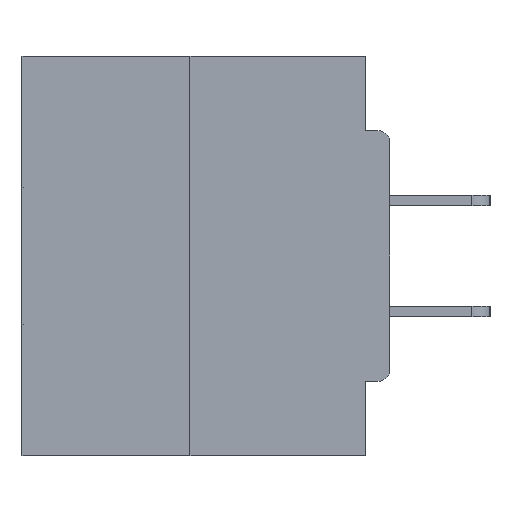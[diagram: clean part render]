
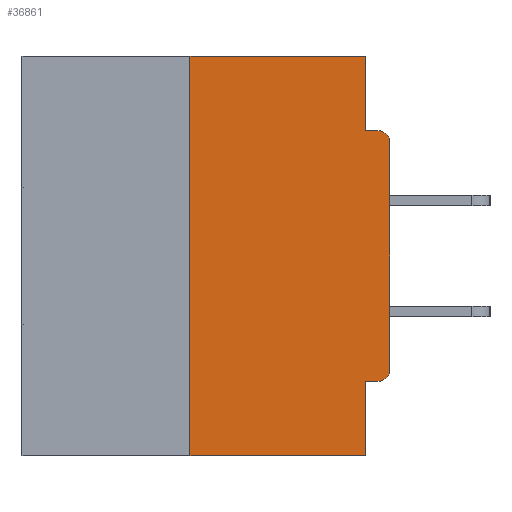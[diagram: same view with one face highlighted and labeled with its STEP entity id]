
A CAD part, left-side view. The second image highlights one B-rep face of the part: STEP entity #36861.
In plain terms, the highlighted planar face has unit normal (-1, 0, 0).
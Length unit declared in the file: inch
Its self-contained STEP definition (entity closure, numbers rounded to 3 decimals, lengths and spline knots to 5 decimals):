
#496 = VECTOR ( 'NONE', #21159, 39.37008 ) ;
#781 = ORIENTED_EDGE ( 'NONE', *, *, #27009, .T. ) ;
#1666 = CARTESIAN_POINT ( 'NONE',  ( 0., 0., 0. ) ) ;
#1993 = CARTESIAN_POINT ( 'NONE',  ( 0., 0.031, 0. ) ) ;
#3010 = VECTOR ( 'NONE', #34634, 39.37008 ) ;
#3475 = PLANE ( 'NONE',  #36398 ) ;
#3596 = AXIS2_PLACEMENT_3D ( 'NONE', #28553, #37429, #28154 ) ;
#4270 = ORIENTED_EDGE ( 'NONE', *, *, #21735, .F. ) ;
#4597 = CARTESIAN_POINT ( 'NONE',  ( 0., 0.031, -0.5 ) ) ;
#4950 = CARTESIAN_POINT ( 'NONE',  ( 0., 0.015, -0.1085 ) ) ;
#5114 = VERTEX_POINT ( 'NONE', #16531 ) ;
#5177 = ORIENTED_EDGE ( 'NONE', *, *, #6664, .F. ) ;
#6664 = EDGE_CURVE ( 'NONE', #37443, #7307, #17230, .T. ) ;
#6822 = DIRECTION ( 'NONE',  ( 0., 0., -1. ) ) ;
#7307 = VERTEX_POINT ( 'NONE', #33008 ) ;
#7712 = ORIENTED_EDGE ( 'NONE', *, *, #18043, .T. ) ;
#7819 = VECTOR ( 'NONE', #20376, 39.37008 ) ;
#7826 = AXIS2_PLACEMENT_3D ( 'NONE', #4950, #31469, #34625 ) ;
#8199 = CARTESIAN_POINT ( 'NONE',  ( 0., 0.25, 0. ) ) ;
#8890 = CARTESIAN_POINT ( 'NONE',  ( 0., 0., -0.0935 ) ) ;
#8992 = LINE ( 'NONE', #33144, #18639 ) ;
#9010 = EDGE_CURVE ( 'NONE', #9735, #37443, #37340, .T. ) ;
#9191 = CARTESIAN_POINT ( 'NONE',  ( 0., 0.46, 0. ) ) ;
#9397 = DIRECTION ( 'NONE',  ( 0., 0., -1. ) ) ;
#9735 = VERTEX_POINT ( 'NONE', #36093 ) ;
#10626 = DIRECTION ( 'NONE',  ( 0., 0., 1. ) ) ;
#10912 = ORIENTED_EDGE ( 'NONE', *, *, #15432, .T. ) ;
#11268 = CARTESIAN_POINT ( 'NONE',  ( 0., 0.46, -0.5 ) ) ;
#12174 = FACE_OUTER_BOUND ( 'NONE', #25087, .T. ) ;
#12441 = LINE ( 'NONE', #8890, #496 ) ;
#12648 = VERTEX_POINT ( 'NONE', #37939 ) ;
#13679 = VECTOR ( 'NONE', #32454, 39.37008 ) ;
#14622 = LINE ( 'NONE', #11268, #7819 ) ;
#14968 = EDGE_CURVE ( 'NONE', #12648, #33162, #8992, .T. ) ;
#15432 = EDGE_CURVE ( 'NONE', #26244, #21813, #21744, .T. ) ;
#15540 = VERTEX_POINT ( 'NONE', #32619 ) ;
#15544 = VERTEX_POINT ( 'NONE', #23908 ) ;
#15575 = CIRCLE ( 'NONE', #3596, 0.015 ) ;
#16531 = CARTESIAN_POINT ( 'NONE',  ( 0., 0.015, -0.4065 ) ) ;
#17198 = CARTESIAN_POINT ( 'NONE',  ( 0., 0.015, -0.0935 ) ) ;
#17230 = LINE ( 'NONE', #19623, #33528 ) ;
#18043 = EDGE_CURVE ( 'NONE', #5114, #15540, #15575, .T. ) ;
#18361 = ORIENTED_EDGE ( 'NONE', *, *, #9010, .F. ) ;
#18639 = VECTOR ( 'NONE', #6822, 39.37008 ) ;
#18725 = ORIENTED_EDGE ( 'NONE', *, *, #29654, .F. ) ;
#18946 = CARTESIAN_POINT ( 'NONE',  ( 0., 0.25, 0. ) ) ;
#19623 = CARTESIAN_POINT ( 'NONE',  ( 0., 0.46, 0. ) ) ;
#20376 = DIRECTION ( 'NONE',  ( 0., -1., 0. ) ) ;
#20426 = LINE ( 'NONE', #1666, #28159 ) ;
#21159 = DIRECTION ( 'NONE',  ( 0., -1., 0. ) ) ;
#21265 = ORIENTED_EDGE ( 'NONE', *, *, #28235, .T. ) ;
#21735 = EDGE_CURVE ( 'NONE', #7307, #15544, #29099, .T. ) ;
#21744 = CIRCLE ( 'NONE', #7826, 0.015 ) ;
#21813 = VERTEX_POINT ( 'NONE', #17198 ) ;
#23908 = CARTESIAN_POINT ( 'NONE',  ( 0., 0.031, -0.0935 ) ) ;
#25087 = EDGE_LOOP ( 'NONE', ( #5177, #18361, #781, #32816, #18725, #7712, #21265, #10912, #27222, #4270 ) ) ;
#26244 = VERTEX_POINT ( 'NONE', #30634 ) ;
#26517 = LINE ( 'NONE', #26708, #13679 ) ;
#26708 = CARTESIAN_POINT ( 'NONE',  ( 0., 0., -0.4065 ) ) ;
#27009 = EDGE_CURVE ( 'NONE', #9735, #33162, #14622, .T. ) ;
#27027 = DIRECTION ( 'NONE',  ( 1., 0., 0. ) ) ;
#27222 = ORIENTED_EDGE ( 'NONE', *, *, #31224, .F. ) ;
#28154 = DIRECTION ( 'NONE',  ( 0., 0., -1. ) ) ;
#28159 = VECTOR ( 'NONE', #34897, 39.37008 ) ;
#28235 = EDGE_CURVE ( 'NONE', #15540, #26244, #20426, .T. ) ;
#28553 = CARTESIAN_POINT ( 'NONE',  ( 0., 0.015, -0.3915 ) ) ;
#29099 = LINE ( 'NONE', #1993, #3010 ) ;
#29311 = DIRECTION ( 'NONE',  ( 0., -1., 0. ) ) ;
#29654 = EDGE_CURVE ( 'NONE', #5114, #12648, #26517, .T. ) ;
#30634 = CARTESIAN_POINT ( 'NONE',  ( 0., 0., -0.1085 ) ) ;
#31224 = EDGE_CURVE ( 'NONE', #15544, #21813, #12441, .T. ) ;
#31469 = DIRECTION ( 'NONE',  ( -1., 0., 0. ) ) ;
#32454 = DIRECTION ( 'NONE',  ( 0., 1., 0. ) ) ;
#32619 = CARTESIAN_POINT ( 'NONE',  ( 0., 0., -0.3915 ) ) ;
#32816 = ORIENTED_EDGE ( 'NONE', *, *, #14968, .F. ) ;
#33008 = CARTESIAN_POINT ( 'NONE',  ( 0., 0.031, 0. ) ) ;
#33144 = CARTESIAN_POINT ( 'NONE',  ( 0., 0.031, -0.5 ) ) ;
#33162 = VERTEX_POINT ( 'NONE', #4597 ) ;
#33528 = VECTOR ( 'NONE', #29311, 39.37008 ) ;
#34625 = DIRECTION ( 'NONE',  ( 0., 0., -1. ) ) ;
#34634 = DIRECTION ( 'NONE',  ( 0., 0., -1. ) ) ;
#34636 = VECTOR ( 'NONE', #10626, 39.37008 ) ;
#34897 = DIRECTION ( 'NONE',  ( 0., 0., 1. ) ) ;
#36093 = CARTESIAN_POINT ( 'NONE',  ( 0., 0.25, -0.5 ) ) ;
#36398 = AXIS2_PLACEMENT_3D ( 'NONE', #9191, #27027, #9397 ) ;
#36861 = ADVANCED_FACE ( 'NONE', ( #12174 ), #3475, .F. ) ;
#37340 = LINE ( 'NONE', #18946, #34636 ) ;
#37429 = DIRECTION ( 'NONE',  ( -1., 0., 0. ) ) ;
#37443 = VERTEX_POINT ( 'NONE', #8199 ) ;
#37939 = CARTESIAN_POINT ( 'NONE',  ( 0., 0.031, -0.4065 ) ) ;
